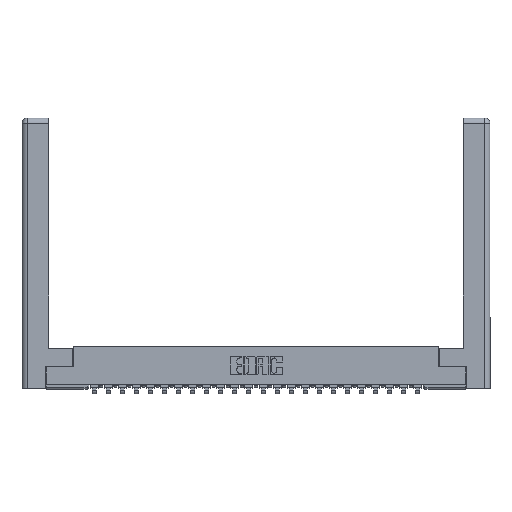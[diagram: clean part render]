
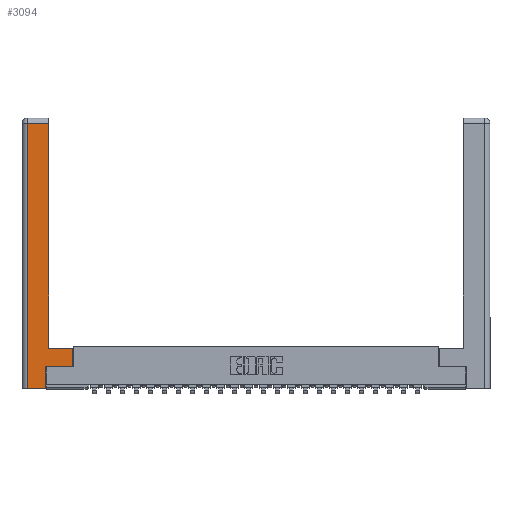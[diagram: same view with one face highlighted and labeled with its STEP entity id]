
A CAD part, top view. The second image highlights one B-rep face of the part: STEP entity #3094.
In plain terms, the highlighted planar face has unit normal (0, 0, 1).
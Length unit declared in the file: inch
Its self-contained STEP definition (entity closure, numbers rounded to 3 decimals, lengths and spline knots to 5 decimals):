
#39 = DIRECTION ( 'NONE',  ( -1., 0., 0. ) ) ;
#202 = VECTOR ( 'NONE', #23056, 39.37008 ) ;
#494 = DIRECTION ( 'NONE',  ( 0., 1., 0. ) ) ;
#2553 = VECTOR ( 'NONE', #21573, 39.37008 ) ;
#2737 = EDGE_CURVE ( 'NONE', #7071, #16174, #22034, .T. ) ;
#2848 = CARTESIAN_POINT ( 'NONE',  ( 0.565, 0.245, 0. ) ) ;
#3013 = EDGE_CURVE ( 'NONE', #3685, #15827, #11096, .T. ) ;
#3094 = ADVANCED_FACE ( 'NONE', ( #13631 ), #25965, .F. ) ;
#3136 = EDGE_CURVE ( 'NONE', #15827, #7071, #12153, .T. ) ;
#3373 = ORIENTED_EDGE ( 'NONE', *, *, #3013, .T. ) ;
#3506 = DIRECTION ( 'NONE',  ( -1., 0., 0. ) ) ;
#3685 = VERTEX_POINT ( 'NONE', #14258 ) ;
#4572 = ORIENTED_EDGE ( 'NONE', *, *, #15490, .T. ) ;
#4777 = ORIENTED_EDGE ( 'NONE', *, *, #2737, .T. ) ;
#5801 = EDGE_LOOP ( 'NONE', ( #4777, #19881, #14961, #4572, #16853, #9963, #3373, #19920 ) ) ;
#6757 = VERTEX_POINT ( 'NONE', #23382 ) ;
#7071 = VERTEX_POINT ( 'NONE', #8340 ) ;
#7477 = CARTESIAN_POINT ( 'NONE',  ( 0.565, 0.45, 0. ) ) ;
#7625 = EDGE_CURVE ( 'NONE', #6757, #20416, #20808, .T. ) ;
#7719 = EDGE_CURVE ( 'NONE', #15694, #16418, #21584, .T. ) ;
#8340 = CARTESIAN_POINT ( 'NONE',  ( 0.295, 0.45, 0. ) ) ;
#9152 = VECTOR ( 'NONE', #21901, 39.37008 ) ;
#9963 = ORIENTED_EDGE ( 'NONE', *, *, #25551, .T. ) ;
#10012 = DIRECTION ( 'NONE',  ( 0., 0., -1. ) ) ;
#10303 = VECTOR ( 'NONE', #494, 39.37008 ) ;
#10703 = CARTESIAN_POINT ( 'NONE',  ( 0.265, 0.245, 0. ) ) ;
#11096 = LINE ( 'NONE', #7477, #10303 ) ;
#11612 = CARTESIAN_POINT ( 'NONE',  ( 0.0615, 0., 0. ) ) ;
#12153 = LINE ( 'NONE', #19857, #12328 ) ;
#12283 = DIRECTION ( 'NONE',  ( -1., 0., 0. ) ) ;
#12328 = VECTOR ( 'NONE', #3506, 39.37008 ) ;
#13055 = CARTESIAN_POINT ( 'NONE',  ( 0.265, 0.245, 0. ) ) ;
#13631 = FACE_OUTER_BOUND ( 'NONE', #5801, .T. ) ;
#14258 = CARTESIAN_POINT ( 'NONE',  ( 0.565, 0.245, 0. ) ) ;
#14780 = CARTESIAN_POINT ( 'NONE',  ( 0.295, 2.94, 0. ) ) ;
#14961 = ORIENTED_EDGE ( 'NONE', *, *, #7719, .T. ) ;
#15478 = VECTOR ( 'NONE', #12283, 39.37008 ) ;
#15490 = EDGE_CURVE ( 'NONE', #16418, #6757, #17361, .T. ) ;
#15624 = CARTESIAN_POINT ( 'NONE',  ( 0.265, 0., 0. ) ) ;
#15694 = VERTEX_POINT ( 'NONE', #24368 ) ;
#15827 = VERTEX_POINT ( 'NONE', #16687 ) ;
#15878 = DIRECTION ( 'NONE',  ( 0., -1., 0. ) ) ;
#15944 = VECTOR ( 'NONE', #15878, 39.37008 ) ;
#16174 = VERTEX_POINT ( 'NONE', #14780 ) ;
#16418 = VERTEX_POINT ( 'NONE', #21396 ) ;
#16687 = CARTESIAN_POINT ( 'NONE',  ( 0.565, 0.45, 0. ) ) ;
#16853 = ORIENTED_EDGE ( 'NONE', *, *, #7625, .T. ) ;
#17361 = LINE ( 'NONE', #15624, #25522 ) ;
#17616 = DIRECTION ( 'NONE',  ( 1., 0., 0. ) ) ;
#18280 = CARTESIAN_POINT ( 'NONE',  ( 0., 0., 0. ) ) ;
#18540 = EDGE_CURVE ( 'NONE', #16174, #15694, #19854, .T. ) ;
#19408 = CARTESIAN_POINT ( 'NONE',  ( 0.295, 3., 0. ) ) ;
#19854 = LINE ( 'NONE', #24101, #15478 ) ;
#19857 = CARTESIAN_POINT ( 'NONE',  ( 0.295, 0.45, 0. ) ) ;
#19881 = ORIENTED_EDGE ( 'NONE', *, *, #18540, .T. ) ;
#19920 = ORIENTED_EDGE ( 'NONE', *, *, #3136, .T. ) ;
#20416 = VERTEX_POINT ( 'NONE', #13055 ) ;
#20808 = LINE ( 'NONE', #10703, #202 ) ;
#21182 = LINE ( 'NONE', #2848, #2553 ) ;
#21396 = CARTESIAN_POINT ( 'NONE',  ( 0.0615, 0., 0. ) ) ;
#21573 = DIRECTION ( 'NONE',  ( 1., 0., 0. ) ) ;
#21584 = LINE ( 'NONE', #11612, #15944 ) ;
#21901 = DIRECTION ( 'NONE',  ( 0., 1., 0. ) ) ;
#22034 = LINE ( 'NONE', #19408, #9152 ) ;
#22602 = AXIS2_PLACEMENT_3D ( 'NONE', #18280, #10012, #39 ) ;
#23056 = DIRECTION ( 'NONE',  ( 0., 1., 0. ) ) ;
#23382 = CARTESIAN_POINT ( 'NONE',  ( 0.265, 0., 0. ) ) ;
#24101 = CARTESIAN_POINT ( 'NONE',  ( 0.0615, 2.94, 0. ) ) ;
#24368 = CARTESIAN_POINT ( 'NONE',  ( 0.0615, 2.94, 0. ) ) ;
#25522 = VECTOR ( 'NONE', #17616, 39.37008 ) ;
#25551 = EDGE_CURVE ( 'NONE', #20416, #3685, #21182, .T. ) ;
#25965 = PLANE ( 'NONE',  #22602 ) ;
